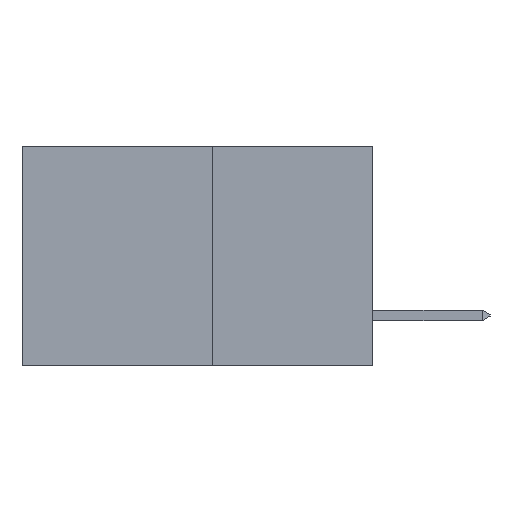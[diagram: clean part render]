
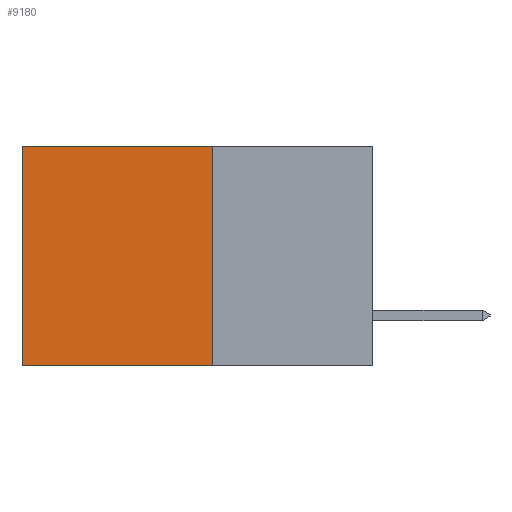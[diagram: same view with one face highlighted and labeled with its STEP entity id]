
A CAD part, left-side view. The second image highlights one B-rep face of the part: STEP entity #9180.
In plain terms, the highlighted planar face has unit normal (-1, 0, 0).
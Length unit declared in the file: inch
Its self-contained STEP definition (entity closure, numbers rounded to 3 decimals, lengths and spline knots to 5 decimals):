
#245 = EDGE_CURVE ( 'NONE', #6224, #14801, #6229, .T. ) ;
#1139 = DIRECTION ( 'NONE',  ( 1., 0., 0. ) ) ;
#1937 = CARTESIAN_POINT ( 'NONE',  ( 0.277, 0.27, -0.37 ) ) ;
#1948 = VERTEX_POINT ( 'NONE', #19054 ) ;
#3848 = CARTESIAN_POINT ( 'NONE',  ( 0.277, 0.27, -0.37 ) ) ;
#5183 = CARTESIAN_POINT ( 'NONE',  ( 0.277, 0.27, 0. ) ) ;
#5934 = LINE ( 'NONE', #10201, #20819 ) ;
#6224 = VERTEX_POINT ( 'NONE', #5183 ) ;
#6229 = LINE ( 'NONE', #14764, #11260 ) ;
#7256 = ORIENTED_EDGE ( 'NONE', *, *, #12947, .F. ) ;
#7741 = EDGE_LOOP ( 'NONE', ( #21529, #7256, #9033, #9677 ) ) ;
#8238 = VECTOR ( 'NONE', #8250, 39.37008 ) ;
#8250 = DIRECTION ( 'NONE',  ( 0., 0., -1. ) ) ;
#9033 = ORIENTED_EDGE ( 'NONE', *, *, #11229, .F. ) ;
#9180 = ADVANCED_FACE ( 'NONE', ( #13633 ), #21705, .F. ) ;
#9677 = ORIENTED_EDGE ( 'NONE', *, *, #245, .T. ) ;
#9714 = EDGE_CURVE ( 'NONE', #14801, #1948, #5934, .T. ) ;
#10201 = CARTESIAN_POINT ( 'NONE',  ( 0.277, 0.59, -0.37 ) ) ;
#11229 = EDGE_CURVE ( 'NONE', #6224, #19837, #23032, .T. ) ;
#11260 = VECTOR ( 'NONE', #23521, 39.37008 ) ;
#12170 = CARTESIAN_POINT ( 'NONE',  ( 0.277, 0.59, 0. ) ) ;
#12515 = CARTESIAN_POINT ( 'NONE',  ( 0.277, 0.27, -0.37 ) ) ;
#12947 = EDGE_CURVE ( 'NONE', #19837, #1948, #14940, .T. ) ;
#13633 = FACE_OUTER_BOUND ( 'NONE', #7741, .T. ) ;
#14433 = DIRECTION ( 'NONE',  ( 0., 0., -1. ) ) ;
#14764 = CARTESIAN_POINT ( 'NONE',  ( 0.277, 0.27, 0. ) ) ;
#14801 = VERTEX_POINT ( 'NONE', #12170 ) ;
#14940 = LINE ( 'NONE', #1937, #23510 ) ;
#18873 = DIRECTION ( 'NONE',  ( 0., 1., 0. ) ) ;
#19054 = CARTESIAN_POINT ( 'NONE',  ( 0.277, 0.59, -0.37 ) ) ;
#19420 = CARTESIAN_POINT ( 'NONE',  ( 0.277, 0.27, -0.37 ) ) ;
#19837 = VERTEX_POINT ( 'NONE', #3848 ) ;
#20819 = VECTOR ( 'NONE', #21284, 39.37008 ) ;
#21284 = DIRECTION ( 'NONE',  ( 0., 0., -1. ) ) ;
#21529 = ORIENTED_EDGE ( 'NONE', *, *, #9714, .T. ) ;
#21705 = PLANE ( 'NONE',  #23496 ) ;
#23032 = LINE ( 'NONE', #19420, #8238 ) ;
#23496 = AXIS2_PLACEMENT_3D ( 'NONE', #12515, #1139, #14433 ) ;
#23510 = VECTOR ( 'NONE', #18873, 39.37008 ) ;
#23521 = DIRECTION ( 'NONE',  ( 0., 1., 0. ) ) ;
